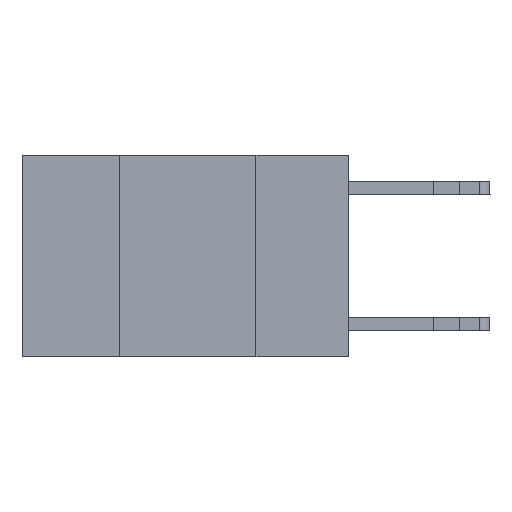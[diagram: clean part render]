
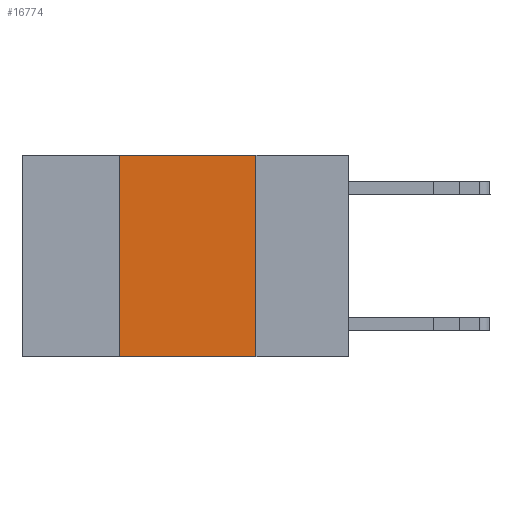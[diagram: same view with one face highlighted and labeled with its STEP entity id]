
A CAD part, left-side view. The second image highlights one B-rep face of the part: STEP entity #16774.
In plain terms, the highlighted planar face has unit normal (-1, 0, 0).
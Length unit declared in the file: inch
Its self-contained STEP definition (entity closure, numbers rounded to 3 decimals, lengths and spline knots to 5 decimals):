
#630 = LINE ( 'NONE', #14949, #11506 ) ;
#1071 = ORIENTED_EDGE ( 'NONE', *, *, #18242, .T. ) ;
#1630 = EDGE_CURVE ( 'NONE', #3659, #9105, #11903, .T. ) ;
#1834 = CARTESIAN_POINT ( 'NONE',  ( 0., 0.17, 0. ) ) ;
#2786 = LINE ( 'NONE', #9174, #12630 ) ;
#3531 = CARTESIAN_POINT ( 'NONE',  ( 0., 0.17, 0. ) ) ;
#3659 = VERTEX_POINT ( 'NONE', #1834 ) ;
#3954 = EDGE_CURVE ( 'NONE', #7416, #8505, #2786, .T. ) ;
#4098 = DIRECTION ( 'NONE',  ( 0., -1., 0. ) ) ;
#4131 = AXIS2_PLACEMENT_3D ( 'NONE', #14245, #12679, #19172 ) ;
#4834 = PLANE ( 'NONE',  #4131 ) ;
#6542 = CARTESIAN_POINT ( 'NONE',  ( 0., 0.17, -0.37 ) ) ;
#6975 = ORIENTED_EDGE ( 'NONE', *, *, #3954, .F. ) ;
#7416 = VERTEX_POINT ( 'NONE', #14689 ) ;
#7994 = EDGE_CURVE ( 'NONE', #8505, #3659, #10692, .T. ) ;
#8287 = ORIENTED_EDGE ( 'NONE', *, *, #1630, .F. ) ;
#8505 = VERTEX_POINT ( 'NONE', #14012 ) ;
#8628 = ORIENTED_EDGE ( 'NONE', *, *, #7994, .F. ) ;
#9105 = VERTEX_POINT ( 'NONE', #6542 ) ;
#9174 = CARTESIAN_POINT ( 'NONE',  ( 0., 0.42, 0. ) ) ;
#10692 = LINE ( 'NONE', #12367, #14263 ) ;
#11506 = VECTOR ( 'NONE', #4098, 39.37008 ) ;
#11903 = LINE ( 'NONE', #3531, #18488 ) ;
#12367 = CARTESIAN_POINT ( 'NONE',  ( 0., 0.6, 0. ) ) ;
#12630 = VECTOR ( 'NONE', #15536, 39.37008 ) ;
#12679 = DIRECTION ( 'NONE',  ( 1., 0., 0. ) ) ;
#14012 = CARTESIAN_POINT ( 'NONE',  ( 0., 0.42, 0. ) ) ;
#14245 = CARTESIAN_POINT ( 'NONE',  ( 0., 0.6, 0. ) ) ;
#14263 = VECTOR ( 'NONE', #20530, 39.37008 ) ;
#14689 = CARTESIAN_POINT ( 'NONE',  ( 0., 0.42, -0.37 ) ) ;
#14949 = CARTESIAN_POINT ( 'NONE',  ( 0., 0.6, -0.37 ) ) ;
#15536 = DIRECTION ( 'NONE',  ( 0., 0., 1. ) ) ;
#16104 = FACE_OUTER_BOUND ( 'NONE', #17757, .T. ) ;
#16273 = DIRECTION ( 'NONE',  ( 0., 0., -1. ) ) ;
#16774 = ADVANCED_FACE ( 'NONE', ( #16104 ), #4834, .F. ) ;
#17757 = EDGE_LOOP ( 'NONE', ( #8287, #8628, #6975, #1071 ) ) ;
#18242 = EDGE_CURVE ( 'NONE', #7416, #9105, #630, .T. ) ;
#18488 = VECTOR ( 'NONE', #16273, 39.37008 ) ;
#19172 = DIRECTION ( 'NONE',  ( 0., 0., -1. ) ) ;
#20530 = DIRECTION ( 'NONE',  ( 0., -1., 0. ) ) ;
